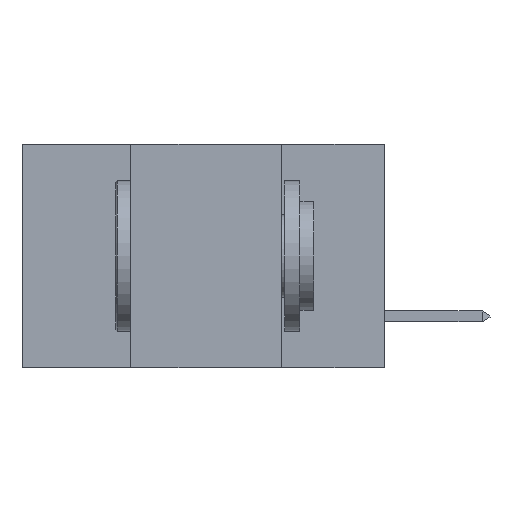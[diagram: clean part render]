
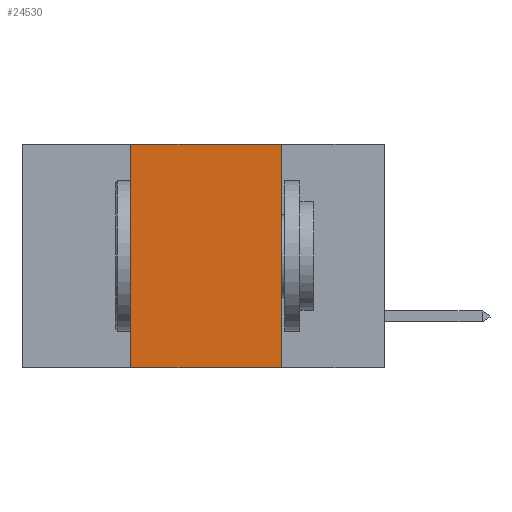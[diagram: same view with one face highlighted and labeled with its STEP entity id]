
A CAD part, left-side view. The second image highlights one B-rep face of the part: STEP entity #24530.
In plain terms, the highlighted planar face has unit normal (-1, 0, 0).
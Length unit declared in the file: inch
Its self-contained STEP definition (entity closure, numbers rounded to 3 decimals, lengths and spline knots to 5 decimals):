
#1383 = VERTEX_POINT ( 'NONE', #6434 ) ;
#1646 = PLANE ( 'NONE',  #15478 ) ;
#4501 = CARTESIAN_POINT ( 'NONE',  ( 0., 0.6, 0. ) ) ;
#4520 = VERTEX_POINT ( 'NONE', #15214 ) ;
#5864 = CARTESIAN_POINT ( 'NONE',  ( 0., 0.42, 0. ) ) ;
#6095 = EDGE_LOOP ( 'NONE', ( #11653, #10547, #22822, #10028 ) ) ;
#6434 = CARTESIAN_POINT ( 'NONE',  ( 0., 0.42, -0.37 ) ) ;
#8323 = DIRECTION ( 'NONE',  ( 0., 0., 1. ) ) ;
#8841 = CARTESIAN_POINT ( 'NONE',  ( 0., 0.6, 0. ) ) ;
#10028 = ORIENTED_EDGE ( 'NONE', *, *, #21829, .T. ) ;
#10390 = LINE ( 'NONE', #17247, #15848 ) ;
#10547 = ORIENTED_EDGE ( 'NONE', *, *, #24013, .F. ) ;
#11041 = EDGE_CURVE ( 'NONE', #4520, #19028, #10390, .T. ) ;
#11175 = DIRECTION ( 'NONE',  ( 1., 0., 0. ) ) ;
#11653 = ORIENTED_EDGE ( 'NONE', *, *, #11041, .F. ) ;
#12409 = LINE ( 'NONE', #22327, #29875 ) ;
#13328 = CARTESIAN_POINT ( 'NONE',  ( 0., 0.17, -0.37 ) ) ;
#15214 = CARTESIAN_POINT ( 'NONE',  ( 0., 0.17, 0. ) ) ;
#15478 = AXIS2_PLACEMENT_3D ( 'NONE', #8841, #11175, #27153 ) ;
#15725 = EDGE_CURVE ( 'NONE', #1383, #21209, #17998, .T. ) ;
#15848 = VECTOR ( 'NONE', #19533, 39.37008 ) ;
#17247 = CARTESIAN_POINT ( 'NONE',  ( 0., 0.17, 0. ) ) ;
#17543 = CARTESIAN_POINT ( 'NONE',  ( 0., 0.42, 0. ) ) ;
#17998 = LINE ( 'NONE', #17543, #29342 ) ;
#18476 = DIRECTION ( 'NONE',  ( 0., -1., 0. ) ) ;
#19028 = VERTEX_POINT ( 'NONE', #13328 ) ;
#19533 = DIRECTION ( 'NONE',  ( 0., 0., -1. ) ) ;
#21209 = VERTEX_POINT ( 'NONE', #5864 ) ;
#21300 = LINE ( 'NONE', #4501, #27308 ) ;
#21829 = EDGE_CURVE ( 'NONE', #1383, #19028, #12409, .T. ) ;
#22327 = CARTESIAN_POINT ( 'NONE',  ( 0., 0.6, -0.37 ) ) ;
#22822 = ORIENTED_EDGE ( 'NONE', *, *, #15725, .F. ) ;
#24013 = EDGE_CURVE ( 'NONE', #21209, #4520, #21300, .T. ) ;
#24530 = ADVANCED_FACE ( 'NONE', ( #24833 ), #1646, .F. ) ;
#24586 = DIRECTION ( 'NONE',  ( 0., -1., 0. ) ) ;
#24833 = FACE_OUTER_BOUND ( 'NONE', #6095, .T. ) ;
#27153 = DIRECTION ( 'NONE',  ( 0., 0., -1. ) ) ;
#27308 = VECTOR ( 'NONE', #18476, 39.37008 ) ;
#29342 = VECTOR ( 'NONE', #8323, 39.37008 ) ;
#29875 = VECTOR ( 'NONE', #24586, 39.37008 ) ;
